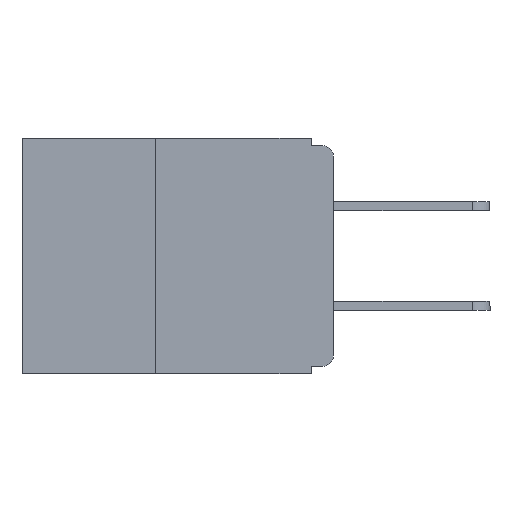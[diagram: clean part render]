
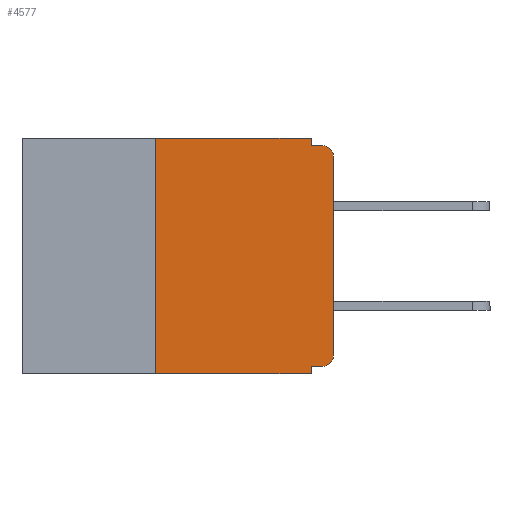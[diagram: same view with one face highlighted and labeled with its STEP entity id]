
A CAD part, left-side view. The second image highlights one B-rep face of the part: STEP entity #4577.
In plain terms, the highlighted planar face has unit normal (-1, 0, 0).
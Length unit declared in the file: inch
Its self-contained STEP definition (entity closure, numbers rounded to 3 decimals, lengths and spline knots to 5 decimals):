
#86 = FACE_OUTER_BOUND ( 'NONE', #13906, .T. ) ;
#168 = ORIENTED_EDGE ( 'NONE', *, *, #15037, .F. ) ;
#169 = VERTEX_POINT ( 'NONE', #10550 ) ;
#227 = CARTESIAN_POINT ( 'NONE',  ( 0., 0.031, -0.01 ) ) ;
#870 = ORIENTED_EDGE ( 'NONE', *, *, #6102, .T. ) ;
#1175 = DIRECTION ( 'NONE',  ( 0., 0., 1. ) ) ;
#1196 = CARTESIAN_POINT ( 'NONE',  ( 0., 0.015, -0.01 ) ) ;
#1206 = CARTESIAN_POINT ( 'NONE',  ( 0., 0.25, -0.33 ) ) ;
#1365 = CARTESIAN_POINT ( 'NONE',  ( 0., 0.015, -0.32 ) ) ;
#1498 = EDGE_CURVE ( 'NONE', #3106, #169, #4011, .T. ) ;
#1610 = EDGE_CURVE ( 'NONE', #1640, #12419, #16518, .T. ) ;
#1640 = VERTEX_POINT ( 'NONE', #1206 ) ;
#1788 = EDGE_CURVE ( 'NONE', #12419, #5707, #18426, .T. ) ;
#1891 = CARTESIAN_POINT ( 'NONE',  ( 0., 0.015, -0.305 ) ) ;
#1997 = VECTOR ( 'NONE', #13732, 39.37008 ) ;
#2621 = VECTOR ( 'NONE', #1175, 39.37008 ) ;
#2656 = CARTESIAN_POINT ( 'NONE',  ( 0., 0.031, 0. ) ) ;
#3102 = LINE ( 'NONE', #10676, #6570 ) ;
#3106 = VERTEX_POINT ( 'NONE', #1365 ) ;
#3351 = ORIENTED_EDGE ( 'NONE', *, *, #11743, .F. ) ;
#3617 = DIRECTION ( 'NONE',  ( 0., -1., 0. ) ) ;
#3825 = CARTESIAN_POINT ( 'NONE',  ( 0., 0., -0.01 ) ) ;
#4011 = CIRCLE ( 'NONE', #11401, 0.015 ) ;
#4021 = ORIENTED_EDGE ( 'NONE', *, *, #9365, .F. ) ;
#4577 = ADVANCED_FACE ( 'NONE', ( #86 ), #12746, .F. ) ;
#4667 = ORIENTED_EDGE ( 'NONE', *, *, #5466, .T. ) ;
#4911 = ORIENTED_EDGE ( 'NONE', *, *, #7546, .F. ) ;
#5430 = VERTEX_POINT ( 'NONE', #7161 ) ;
#5466 = EDGE_CURVE ( 'NONE', #12930, #14616, #7975, .T. ) ;
#5707 = VERTEX_POINT ( 'NONE', #2656 ) ;
#5890 = ORIENTED_EDGE ( 'NONE', *, *, #1498, .T. ) ;
#6102 = EDGE_CURVE ( 'NONE', #169, #12930, #18485, .T. ) ;
#6570 = VECTOR ( 'NONE', #10588, 39.37008 ) ;
#6595 = DIRECTION ( 'NONE',  ( 0., 0., -1. ) ) ;
#6620 = DIRECTION ( 'NONE',  ( -1., 0., 0. ) ) ;
#6625 = CARTESIAN_POINT ( 'NONE',  ( 0., 0.015, -0.025 ) ) ;
#7161 = CARTESIAN_POINT ( 'NONE',  ( 0., 0.031, -0.33 ) ) ;
#7482 = DIRECTION ( 'NONE',  ( -1., 0., 0. ) ) ;
#7546 = EDGE_CURVE ( 'NONE', #5707, #8695, #3102, .T. ) ;
#7835 = DIRECTION ( 'NONE',  ( 0., 0., -1. ) ) ;
#7975 = CIRCLE ( 'NONE', #10610, 0.015 ) ;
#8654 = DIRECTION ( 'NONE',  ( 0., 0., -1. ) ) ;
#8695 = VERTEX_POINT ( 'NONE', #227 ) ;
#9246 = ORIENTED_EDGE ( 'NONE', *, *, #1788, .F. ) ;
#9365 = EDGE_CURVE ( 'NONE', #3106, #16777, #17640, .T. ) ;
#10550 = CARTESIAN_POINT ( 'NONE',  ( 0., 0., -0.305 ) ) ;
#10588 = DIRECTION ( 'NONE',  ( 0., 0., -1. ) ) ;
#10610 = AXIS2_PLACEMENT_3D ( 'NONE', #6625, #6620, #6595 ) ;
#10662 = DIRECTION ( 'NONE',  ( 0., -1., 0. ) ) ;
#10676 = CARTESIAN_POINT ( 'NONE',  ( 0., 0.031, 0. ) ) ;
#10686 = CARTESIAN_POINT ( 'NONE',  ( 0., 0.437, 0. ) ) ;
#10893 = CARTESIAN_POINT ( 'NONE',  ( 0., 0., -0.32 ) ) ;
#11331 = VECTOR ( 'NONE', #13913, 39.37008 ) ;
#11401 = AXIS2_PLACEMENT_3D ( 'NONE', #1891, #7482, #8654 ) ;
#11461 = LINE ( 'NONE', #16309, #12385 ) ;
#11612 = CARTESIAN_POINT ( 'NONE',  ( 0., 0., -0.025 ) ) ;
#11738 = ORIENTED_EDGE ( 'NONE', *, *, #15496, .T. ) ;
#11743 = EDGE_CURVE ( 'NONE', #16777, #5430, #11461, .T. ) ;
#11963 = CARTESIAN_POINT ( 'NONE',  ( 0., 0.25, 0. ) ) ;
#12106 = DIRECTION ( 'NONE',  ( 0., 0., -1. ) ) ;
#12318 = DIRECTION ( 'NONE',  ( 1., 0., 0. ) ) ;
#12339 = CARTESIAN_POINT ( 'NONE',  ( 0., 0.437, -0.33 ) ) ;
#12360 = CARTESIAN_POINT ( 'NONE',  ( 0., 0.031, -0.32 ) ) ;
#12385 = VECTOR ( 'NONE', #7835, 39.37008 ) ;
#12419 = VERTEX_POINT ( 'NONE', #11963 ) ;
#12546 = CARTESIAN_POINT ( 'NONE',  ( 0., 0.437, 0. ) ) ;
#12746 = PLANE ( 'NONE',  #18171 ) ;
#12851 = ORIENTED_EDGE ( 'NONE', *, *, #1610, .F. ) ;
#12930 = VERTEX_POINT ( 'NONE', #11612 ) ;
#13562 = CARTESIAN_POINT ( 'NONE',  ( 0., 0., 0. ) ) ;
#13579 = DIRECTION ( 'NONE',  ( 0., 0., 1. ) ) ;
#13732 = DIRECTION ( 'NONE',  ( 0., 1., 0. ) ) ;
#13906 = EDGE_LOOP ( 'NONE', ( #870, #4667, #168, #4911, #9246, #12851, #11738, #3351, #4021, #5890 ) ) ;
#13913 = DIRECTION ( 'NONE',  ( 0., -1., 0. ) ) ;
#14616 = VERTEX_POINT ( 'NONE', #1196 ) ;
#14851 = VECTOR ( 'NONE', #13579, 39.37008 ) ;
#15036 = VECTOR ( 'NONE', #3617, 39.37008 ) ;
#15037 = EDGE_CURVE ( 'NONE', #8695, #14616, #15053, .T. ) ;
#15053 = LINE ( 'NONE', #3825, #11331 ) ;
#15496 = EDGE_CURVE ( 'NONE', #1640, #5430, #18262, .T. ) ;
#16309 = CARTESIAN_POINT ( 'NONE',  ( 0., 0.031, -0.33 ) ) ;
#16518 = LINE ( 'NONE', #16676, #2621 ) ;
#16676 = CARTESIAN_POINT ( 'NONE',  ( 0., 0.25, -0.33 ) ) ;
#16777 = VERTEX_POINT ( 'NONE', #12360 ) ;
#17572 = VECTOR ( 'NONE', #10662, 39.37008 ) ;
#17640 = LINE ( 'NONE', #10893, #1997 ) ;
#18171 = AXIS2_PLACEMENT_3D ( 'NONE', #12546, #12318, #12106 ) ;
#18262 = LINE ( 'NONE', #12339, #15036 ) ;
#18426 = LINE ( 'NONE', #10686, #17572 ) ;
#18485 = LINE ( 'NONE', #13562, #14851 ) ;
